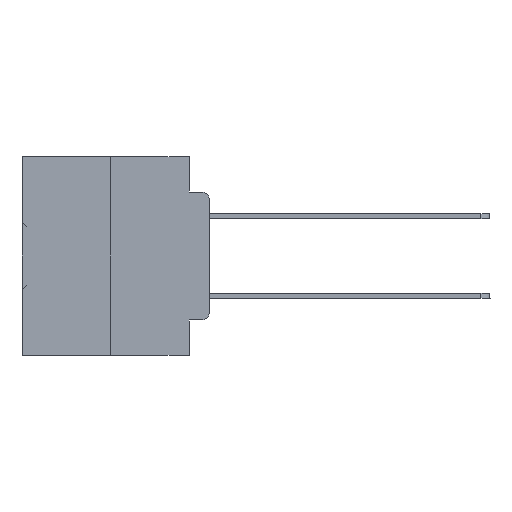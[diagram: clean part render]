
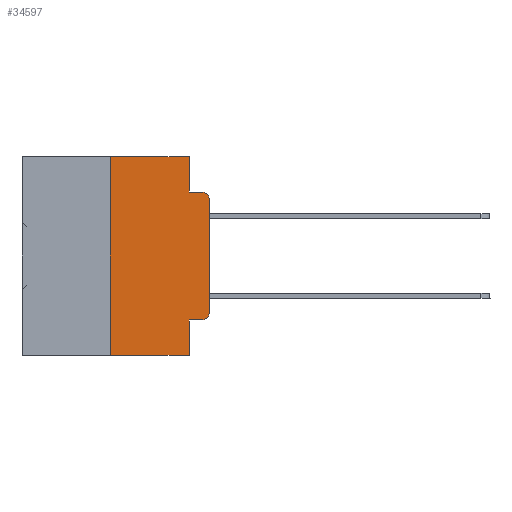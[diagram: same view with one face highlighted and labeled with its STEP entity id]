
A CAD part, left-side view. The second image highlights one B-rep face of the part: STEP entity #34597.
In plain terms, the highlighted planar face has unit normal (-1, 0, 0).
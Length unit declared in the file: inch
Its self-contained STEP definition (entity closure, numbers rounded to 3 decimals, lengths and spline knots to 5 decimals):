
#790 = DIRECTION ( 'NONE',  ( 0., 0., -1. ) ) ;
#1105 = DIRECTION ( 'NONE',  ( 0., 0., -1. ) ) ;
#1415 = CARTESIAN_POINT ( 'NONE',  ( 0., 0.051, -0.5 ) ) ;
#2187 = LINE ( 'NONE', #39080, #28766 ) ;
#2750 = ORIENTED_EDGE ( 'NONE', *, *, #24505, .F. ) ;
#3348 = DIRECTION ( 'NONE',  ( -1., 0., 0. ) ) ;
#3601 = EDGE_CURVE ( 'NONE', #35091, #22125, #25424, .T. ) ;
#4264 = VERTEX_POINT ( 'NONE', #8785 ) ;
#5187 = LINE ( 'NONE', #20377, #24125 ) ;
#5568 = AXIS2_PLACEMENT_3D ( 'NONE', #11572, #23911, #17864 ) ;
#6381 = CARTESIAN_POINT ( 'NONE',  ( 0., 0., -0.1085 ) ) ;
#7664 = EDGE_CURVE ( 'NONE', #20118, #16644, #2187, .T. ) ;
#7943 = PLANE ( 'NONE',  #5568 ) ;
#7963 = VECTOR ( 'NONE', #20933, 39.37008 ) ;
#8095 = EDGE_CURVE ( 'NONE', #16644, #28854, #26127, .T. ) ;
#8785 = CARTESIAN_POINT ( 'NONE',  ( 0., 0.02, -0.0885 ) ) ;
#9052 = EDGE_CURVE ( 'NONE', #10533, #22125, #5187, .T. ) ;
#9187 = LINE ( 'NONE', #14854, #7963 ) ;
#9246 = VECTOR ( 'NONE', #13792, 39.37008 ) ;
#9470 = DIRECTION ( 'NONE',  ( 0., 0., -1. ) ) ;
#9843 = VERTEX_POINT ( 'NONE', #30833 ) ;
#10040 = EDGE_CURVE ( 'NONE', #9843, #21483, #10551, .T. ) ;
#10533 = VERTEX_POINT ( 'NONE', #39611 ) ;
#10551 = LINE ( 'NONE', #35464, #9246 ) ;
#10889 = ORIENTED_EDGE ( 'NONE', *, *, #34293, .F. ) ;
#10930 = DIRECTION ( 'NONE',  ( -1., 0., 0. ) ) ;
#11496 = EDGE_LOOP ( 'NONE', ( #13527, #27762, #10889, #36147, #35446, #2750, #39661, #21801, #18262, #27448 ) ) ;
#11572 = CARTESIAN_POINT ( 'NONE',  ( 0., 0.473, 0. ) ) ;
#11808 = AXIS2_PLACEMENT_3D ( 'NONE', #16311, #3348, #9470 ) ;
#11861 = EDGE_CURVE ( 'NONE', #21483, #4264, #34431, .T. ) ;
#13527 = ORIENTED_EDGE ( 'NONE', *, *, #10040, .T. ) ;
#13780 = CIRCLE ( 'NONE', #27362, 0.02 ) ;
#13792 = DIRECTION ( 'NONE',  ( 0., 0., 1. ) ) ;
#14854 = CARTESIAN_POINT ( 'NONE',  ( 0., 0.051, -0.4115 ) ) ;
#14886 = CARTESIAN_POINT ( 'NONE',  ( 0., 0.051, 0. ) ) ;
#16311 = CARTESIAN_POINT ( 'NONE',  ( 0., 0.02, -0.1085 ) ) ;
#16644 = VERTEX_POINT ( 'NONE', #14886 ) ;
#17778 = CARTESIAN_POINT ( 'NONE',  ( 0., 0.02, -0.4115 ) ) ;
#17864 = DIRECTION ( 'NONE',  ( 0., 0., -1. ) ) ;
#18134 = CARTESIAN_POINT ( 'NONE',  ( 0., 0.051, -0.0885 ) ) ;
#18262 = ORIENTED_EDGE ( 'NONE', *, *, #32065, .T. ) ;
#19544 = CARTESIAN_POINT ( 'NONE',  ( 0., 0.051, 0. ) ) ;
#20118 = VERTEX_POINT ( 'NONE', #20496 ) ;
#20377 = CARTESIAN_POINT ( 'NONE',  ( 0., 0.473, -0.5 ) ) ;
#20455 = DIRECTION ( 'NONE',  ( 0., 0., -1. ) ) ;
#20496 = CARTESIAN_POINT ( 'NONE',  ( 0., 0.25, 0. ) ) ;
#20634 = CARTESIAN_POINT ( 'NONE',  ( 0., 0.02, -0.3915 ) ) ;
#20674 = FACE_OUTER_BOUND ( 'NONE', #11496, .T. ) ;
#20933 = DIRECTION ( 'NONE',  ( 0., -1., 0. ) ) ;
#21090 = VECTOR ( 'NONE', #39250, 39.37008 ) ;
#21483 = VERTEX_POINT ( 'NONE', #6381 ) ;
#21801 = ORIENTED_EDGE ( 'NONE', *, *, #3601, .F. ) ;
#22125 = VERTEX_POINT ( 'NONE', #1415 ) ;
#22904 = CARTESIAN_POINT ( 'NONE',  ( 0., 0.051, 0. ) ) ;
#23208 = DIRECTION ( 'NONE',  ( 0., -1., 0. ) ) ;
#23911 = DIRECTION ( 'NONE',  ( 1., 0., 0. ) ) ;
#24125 = VECTOR ( 'NONE', #23208, 39.37008 ) ;
#24505 = EDGE_CURVE ( 'NONE', #10533, #20118, #32948, .T. ) ;
#25212 = VECTOR ( 'NONE', #1105, 39.37008 ) ;
#25424 = LINE ( 'NONE', #19544, #25212 ) ;
#26127 = LINE ( 'NONE', #22904, #36567 ) ;
#26874 = CARTESIAN_POINT ( 'NONE',  ( 0., 0.25, 0. ) ) ;
#27362 = AXIS2_PLACEMENT_3D ( 'NONE', #20634, #10930, #20455 ) ;
#27448 = ORIENTED_EDGE ( 'NONE', *, *, #32355, .T. ) ;
#27762 = ORIENTED_EDGE ( 'NONE', *, *, #11861, .T. ) ;
#28766 = VECTOR ( 'NONE', #32585, 39.37008 ) ;
#28854 = VERTEX_POINT ( 'NONE', #38571 ) ;
#29448 = VECTOR ( 'NONE', #30292, 39.37008 ) ;
#30292 = DIRECTION ( 'NONE',  ( 0., -1., 0. ) ) ;
#30833 = CARTESIAN_POINT ( 'NONE',  ( 0., 0., -0.3915 ) ) ;
#32065 = EDGE_CURVE ( 'NONE', #35091, #39241, #9187, .T. ) ;
#32355 = EDGE_CURVE ( 'NONE', #39241, #9843, #13780, .T. ) ;
#32585 = DIRECTION ( 'NONE',  ( 0., -1., 0. ) ) ;
#32948 = LINE ( 'NONE', #26874, #21090 ) ;
#34293 = EDGE_CURVE ( 'NONE', #28854, #4264, #37169, .T. ) ;
#34431 = CIRCLE ( 'NONE', #11808, 0.02 ) ;
#34597 = ADVANCED_FACE ( 'NONE', ( #20674 ), #7943, .F. ) ;
#35091 = VERTEX_POINT ( 'NONE', #39679 ) ;
#35446 = ORIENTED_EDGE ( 'NONE', *, *, #7664, .F. ) ;
#35464 = CARTESIAN_POINT ( 'NONE',  ( 0., 0., 0. ) ) ;
#36147 = ORIENTED_EDGE ( 'NONE', *, *, #8095, .F. ) ;
#36567 = VECTOR ( 'NONE', #790, 39.37008 ) ;
#37169 = LINE ( 'NONE', #18134, #29448 ) ;
#38571 = CARTESIAN_POINT ( 'NONE',  ( 0., 0.051, -0.0885 ) ) ;
#39080 = CARTESIAN_POINT ( 'NONE',  ( 0., 0.473, 0. ) ) ;
#39241 = VERTEX_POINT ( 'NONE', #17778 ) ;
#39250 = DIRECTION ( 'NONE',  ( 0., 0., 1. ) ) ;
#39611 = CARTESIAN_POINT ( 'NONE',  ( 0., 0.25, -0.5 ) ) ;
#39661 = ORIENTED_EDGE ( 'NONE', *, *, #9052, .T. ) ;
#39679 = CARTESIAN_POINT ( 'NONE',  ( 0., 0.051, -0.4115 ) ) ;
